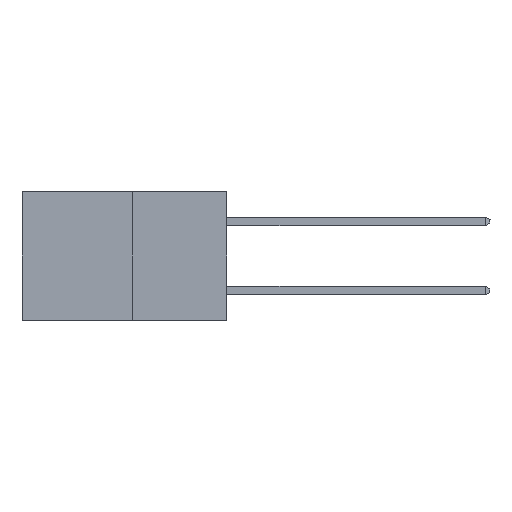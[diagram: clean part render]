
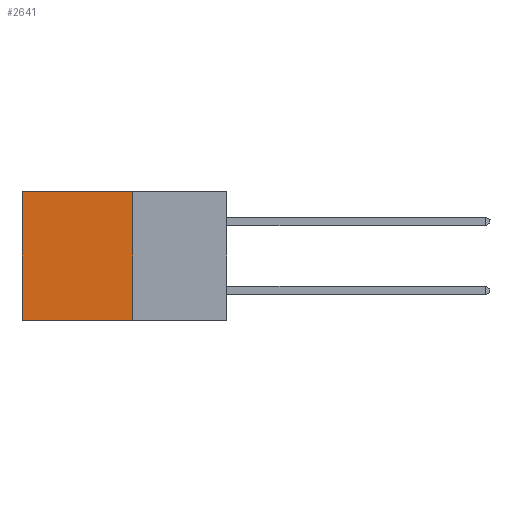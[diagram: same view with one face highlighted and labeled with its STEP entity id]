
A CAD part, left-side view. The second image highlights one B-rep face of the part: STEP entity #2641.
In plain terms, the highlighted planar face has unit normal (-1, 0, 0).
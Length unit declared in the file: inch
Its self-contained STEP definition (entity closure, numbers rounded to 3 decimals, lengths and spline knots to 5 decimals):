
#1272 = DIRECTION ( 'NONE',  ( 0., 1., 0. ) ) ;
#1561 = DIRECTION ( 'NONE',  ( 1., 0., 0. ) ) ;
#1873 = EDGE_CURVE ( 'NONE', #11727, #5420, #15151, .T. ) ;
#2529 = ORIENTED_EDGE ( 'NONE', *, *, #1873, .T. ) ;
#2641 = ADVANCED_FACE ( 'NONE', ( #10940 ), #8944, .F. ) ;
#2656 = LINE ( 'NONE', #11378, #8838 ) ;
#3699 = ORIENTED_EDGE ( 'NONE', *, *, #7642, .F. ) ;
#4277 = CARTESIAN_POINT ( 'NONE',  ( 0.277, 0.59, -0.37 ) ) ;
#5031 = DIRECTION ( 'NONE',  ( 0., 0., -1. ) ) ;
#5259 = VECTOR ( 'NONE', #1272, 39.37008 ) ;
#5420 = VERTEX_POINT ( 'NONE', #8746 ) ;
#5533 = DIRECTION ( 'NONE',  ( 0., 1., 0. ) ) ;
#5673 = CARTESIAN_POINT ( 'NONE',  ( 0.277, 0.27, -0.37 ) ) ;
#6670 = LINE ( 'NONE', #6714, #13333 ) ;
#6714 = CARTESIAN_POINT ( 'NONE',  ( 0.277, 0.27, -0.37 ) ) ;
#7235 = LINE ( 'NONE', #9279, #10589 ) ;
#7642 = EDGE_CURVE ( 'NONE', #10419, #14755, #7235, .T. ) ;
#8143 = ORIENTED_EDGE ( 'NONE', *, *, #15795, .T. ) ;
#8351 = ORIENTED_EDGE ( 'NONE', *, *, #12094, .F. ) ;
#8746 = CARTESIAN_POINT ( 'NONE',  ( 0.277, 0.59, 0. ) ) ;
#8838 = VECTOR ( 'NONE', #12612, 39.37008 ) ;
#8944 = PLANE ( 'NONE',  #13270 ) ;
#9279 = CARTESIAN_POINT ( 'NONE',  ( 0.277, 0.27, -0.37 ) ) ;
#9713 = CARTESIAN_POINT ( 'NONE',  ( 0.277, 0.27, 0. ) ) ;
#10419 = VERTEX_POINT ( 'NONE', #15598 ) ;
#10589 = VECTOR ( 'NONE', #5533, 39.37008 ) ;
#10940 = FACE_OUTER_BOUND ( 'NONE', #12199, .T. ) ;
#11378 = CARTESIAN_POINT ( 'NONE',  ( 0.277, 0.59, -0.37 ) ) ;
#11727 = VERTEX_POINT ( 'NONE', #9713 ) ;
#12094 = EDGE_CURVE ( 'NONE', #11727, #10419, #6670, .T. ) ;
#12199 = EDGE_LOOP ( 'NONE', ( #8143, #3699, #8351, #2529 ) ) ;
#12612 = DIRECTION ( 'NONE',  ( 0., 0., -1. ) ) ;
#13270 = AXIS2_PLACEMENT_3D ( 'NONE', #5673, #1561, #5031 ) ;
#13333 = VECTOR ( 'NONE', #15348, 39.37008 ) ;
#14755 = VERTEX_POINT ( 'NONE', #4277 ) ;
#14772 = CARTESIAN_POINT ( 'NONE',  ( 0.277, 0.27, 0. ) ) ;
#15151 = LINE ( 'NONE', #14772, #5259 ) ;
#15348 = DIRECTION ( 'NONE',  ( 0., 0., -1. ) ) ;
#15598 = CARTESIAN_POINT ( 'NONE',  ( 0.277, 0.27, -0.37 ) ) ;
#15795 = EDGE_CURVE ( 'NONE', #5420, #14755, #2656, .T. ) ;
